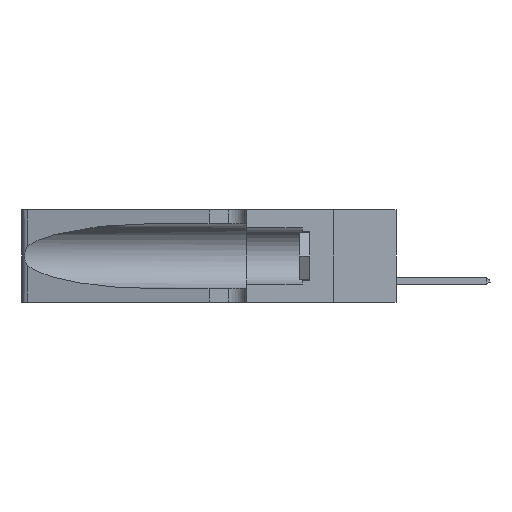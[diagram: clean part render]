
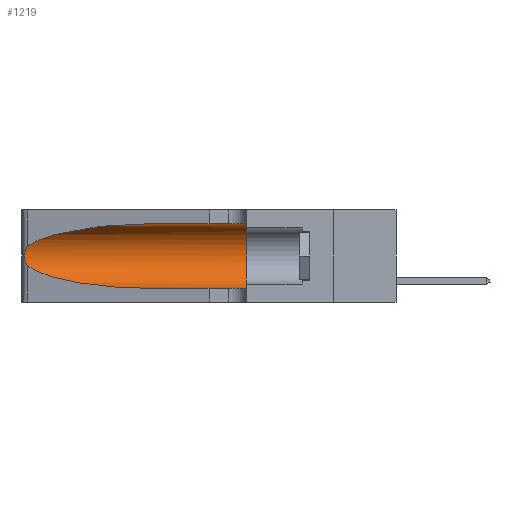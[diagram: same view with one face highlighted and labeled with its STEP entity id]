
A CAD part, left-side view. The second image highlights one B-rep face of the part: STEP entity #1219.
In plain terms, the highlighted cylindrical face has radius 3.308 mm (diameter 6.617 mm), a partial arc.
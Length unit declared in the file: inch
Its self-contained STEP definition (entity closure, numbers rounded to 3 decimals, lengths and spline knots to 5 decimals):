
#1219 = ADVANCED_FACE ( 'NONE', ( #20571 ), #25977, .F. ) ;
#1605 = B_SPLINE_CURVE_WITH_KNOTS ( 'NONE', 3,
 ( #7586, #23719, #10366, #10023, #31387, #5057, #28933, #18385, #34104, #2603, #18173, #28820, #7365, #2508 ),
 .UNSPECIFIED., .F., .F.,
 ( 4, 2, 2, 2, 2, 2, 4 ),
 ( 0., 0.00027, 0.00053, 0.00107, 0.0016, 0.00187, 0.00214 ),
 .UNSPECIFIED. ) ;
#2300 = DIRECTION ( 'NONE',  ( 0., 1., 0. ) ) ;
#2508 = CARTESIAN_POINT ( 'NONE',  ( 0.25487, 1.22718, 0.14631 ) ) ;
#2603 = CARTESIAN_POINT ( 'NONE',  ( 0.25856, 1.23593, 0.16098 ) ) ;
#2772 = EDGE_CURVE ( 'NONE', #32669, #20437, #18565, .T. ) ;
#2901 = CARTESIAN_POINT ( 'NONE',  ( 0.18966, 0.96281, 0.05475 ) ) ;
#3782 = VECTOR ( 'NONE', #20260, 39.37008 ) ;
#4160 = EDGE_CURVE ( 'NONE', #4166, #21086, #10780, .T. ) ;
#4166 = VERTEX_POINT ( 'NONE', #26755 ) ;
#5057 = CARTESIAN_POINT ( 'NONE',  ( 0.26018, 1.23835, 0.19895 ) ) ;
#6440 = ORIENTED_EDGE ( 'NONE', *, *, #7544, .T. ) ;
#7083 = LINE ( 'NONE', #17594, #3782 ) ;
#7365 = CARTESIAN_POINT ( 'NONE',  ( 0.25555, 1.22993, 0.14849 ) ) ;
#7544 = EDGE_CURVE ( 'NONE', #21086, #30918, #7083, .T. ) ;
#7586 = CARTESIAN_POINT ( 'NONE',  ( 0.25487, 1.22718, 0.22369 ) ) ;
#7736 = ORIENTED_EDGE ( 'NONE', *, *, #22059, .F. ) ;
#10023 = CARTESIAN_POINT ( 'NONE',  ( 0.25787, 1.23484, 0.2124 ) ) ;
#10366 = CARTESIAN_POINT ( 'NONE',  ( 0.25639, 1.23184, 0.21858 ) ) ;
#10647 = ORIENTED_EDGE ( 'NONE', *, *, #2772, .F. ) ;
#10780 =( BOUNDED_CURVE ( )  B_SPLINE_CURVE ( 3, ( #21893, #13628, #2901, #18855 ),
 .UNSPECIFIED., .F., .T. ) 
 B_SPLINE_CURVE_WITH_KNOTS ( ( 4, 4 ),
 ( 3.44316, 4.71239 ),
 .UNSPECIFIED. ) 
 CURVE ( )  GEOMETRIC_REPRESENTATION_ITEM ( )  RATIONAL_B_SPLINE_CURVE ( ( 1., 0.87, 0.87, 1. ) ) 
 REPRESENTATION_ITEM ( '' )  );
#12808 = CARTESIAN_POINT ( 'NONE',  ( 0.2373, 1.15595, 0.28018 ) ) ;
#12934 = DIRECTION ( 'NONE',  ( 0., 0., 1. ) ) ;
#13628 = CARTESIAN_POINT ( 'NONE',  ( 0.2373, 1.15595, 0.08982 ) ) ;
#14370 = AXIS2_PLACEMENT_3D ( 'NONE', #16780, #24682, #32483 ) ;
#14979 =( BOUNDED_CURVE ( )  B_SPLINE_CURVE ( 3, ( #33992, #28715, #12808, #31620 ),
 .UNSPECIFIED., .F., .T. ) 
 B_SPLINE_CURVE_WITH_KNOTS ( ( 4, 4 ),
 ( 1.5708, 2.84003 ),
 .UNSPECIFIED. ) 
 CURVE ( )  GEOMETRIC_REPRESENTATION_ITEM ( )  RATIONAL_B_SPLINE_CURVE ( ( 1., 0.87, 0.87, 1. ) ) 
 REPRESENTATION_ITEM ( '' )  );
#15494 = CARTESIAN_POINT ( 'NONE',  ( 0.1305, 0.35, 0.185 ) ) ;
#16301 = CARTESIAN_POINT ( 'NONE',  ( 0.1305, 0.35, 0.31525 ) ) ;
#16317 = CARTESIAN_POINT ( 'NONE',  ( 0.1305, 0.72297, 0.05475 ) ) ;
#16434 = ORIENTED_EDGE ( 'NONE', *, *, #29139, .T. ) ;
#16780 = CARTESIAN_POINT ( 'NONE',  ( 0.1305, 1.61858, 0.185 ) ) ;
#17421 = CIRCLE ( 'NONE', #23961, 0.13025 ) ;
#17594 = CARTESIAN_POINT ( 'NONE',  ( 0.1305, 1.61858, 0.05475 ) ) ;
#18173 = CARTESIAN_POINT ( 'NONE',  ( 0.25789, 1.23486, 0.15765 ) ) ;
#18385 = CARTESIAN_POINT ( 'NONE',  ( 0.26075, 1.23896, 0.178 ) ) ;
#18565 = LINE ( 'NONE', #20422, #29335 ) ;
#18684 = ORIENTED_EDGE ( 'NONE', *, *, #29158, .T. ) ;
#18855 = CARTESIAN_POINT ( 'NONE',  ( 0.1305, 0.72297, 0.05475 ) ) ;
#20260 = DIRECTION ( 'NONE',  ( 0., -1., 0. ) ) ;
#20422 = CARTESIAN_POINT ( 'NONE',  ( 0.1305, 1.61858, 0.31525 ) ) ;
#20437 = VERTEX_POINT ( 'NONE', #16301 ) ;
#20571 = FACE_OUTER_BOUND ( 'NONE', #31372, .T. ) ;
#21086 = VERTEX_POINT ( 'NONE', #16317 ) ;
#21893 = CARTESIAN_POINT ( 'NONE',  ( 0.25487, 1.22718, 0.14631 ) ) ;
#22059 = EDGE_CURVE ( 'NONE', #20437, #30918, #17421, .T. ) ;
#22996 = ORIENTED_EDGE ( 'NONE', *, *, #4160, .T. ) ;
#23065 = CARTESIAN_POINT ( 'NONE',  ( 0.25487, 1.22718, 0.22369 ) ) ;
#23719 = CARTESIAN_POINT ( 'NONE',  ( 0.25555, 1.22994, 0.2215 ) ) ;
#23961 = AXIS2_PLACEMENT_3D ( 'NONE', #15494, #2300, #12934 ) ;
#24682 = DIRECTION ( 'NONE',  ( 0., -1., 0. ) ) ;
#25977 = CYLINDRICAL_SURFACE ( 'NONE', #14370, 0.13025 ) ;
#26755 = CARTESIAN_POINT ( 'NONE',  ( 0.25487, 1.22718, 0.14631 ) ) ;
#27028 = CARTESIAN_POINT ( 'NONE',  ( 0.1305, 0.35, 0.05475 ) ) ;
#28667 = DIRECTION ( 'NONE',  ( 0., -1., 0. ) ) ;
#28715 = CARTESIAN_POINT ( 'NONE',  ( 0.18966, 0.96281, 0.31525 ) ) ;
#28820 = CARTESIAN_POINT ( 'NONE',  ( 0.25639, 1.23186, 0.15144 ) ) ;
#28933 = CARTESIAN_POINT ( 'NONE',  ( 0.26075, 1.23896, 0.19203 ) ) ;
#29139 = EDGE_CURVE ( 'NONE', #32669, #33664, #14979, .T. ) ;
#29158 = EDGE_CURVE ( 'NONE', #33664, #4166, #1605, .T. ) ;
#29335 = VECTOR ( 'NONE', #28667, 39.37008 ) ;
#29686 = CARTESIAN_POINT ( 'NONE',  ( 0.1305, 0.72297, 0.31525 ) ) ;
#30918 = VERTEX_POINT ( 'NONE', #27028 ) ;
#31372 = EDGE_LOOP ( 'NONE', ( #16434, #18684, #22996, #6440, #7736, #10647 ) ) ;
#31387 = CARTESIAN_POINT ( 'NONE',  ( 0.25854, 1.2359, 0.20912 ) ) ;
#31620 = CARTESIAN_POINT ( 'NONE',  ( 0.25487, 1.22718, 0.22369 ) ) ;
#32483 = DIRECTION ( 'NONE',  ( 0., 0., -1. ) ) ;
#32669 = VERTEX_POINT ( 'NONE', #29686 ) ;
#33664 = VERTEX_POINT ( 'NONE', #23065 ) ;
#33992 = CARTESIAN_POINT ( 'NONE',  ( 0.1305, 0.72297, 0.31525 ) ) ;
#34104 = CARTESIAN_POINT ( 'NONE',  ( 0.26017, 1.23833, 0.17102 ) ) ;
